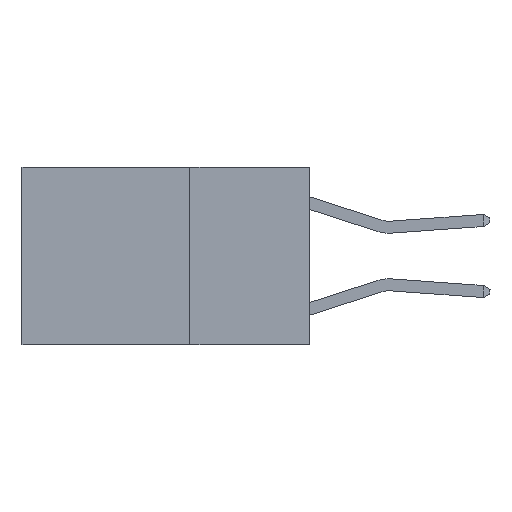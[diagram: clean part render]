
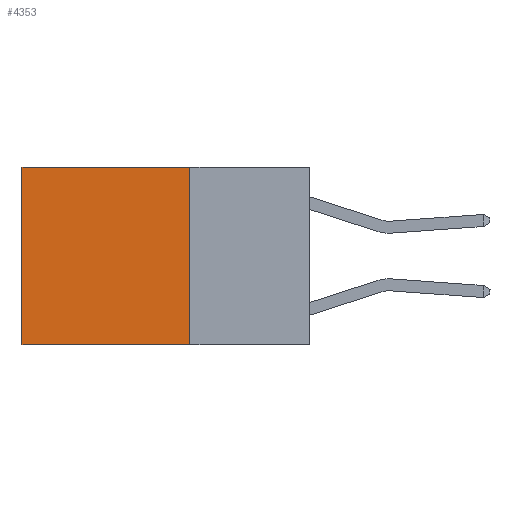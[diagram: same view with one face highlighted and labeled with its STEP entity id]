
A CAD part, left-side view. The second image highlights one B-rep face of the part: STEP entity #4353.
In plain terms, the highlighted planar face has unit normal (-1, 0, 0).
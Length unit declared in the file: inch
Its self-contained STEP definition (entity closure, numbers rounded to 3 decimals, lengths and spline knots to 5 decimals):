
#107 = EDGE_CURVE ( 'NONE', #16275, #7895, #18530, .T. ) ;
#217 = LINE ( 'NONE', #10510, #25759 ) ;
#487 = DIRECTION ( 'NONE',  ( 0., 0., -1. ) ) ;
#1403 = LINE ( 'NONE', #7564, #20456 ) ;
#2352 = CARTESIAN_POINT ( 'NONE',  ( 0.2625, 0.6, 0. ) ) ;
#2807 = PLANE ( 'NONE',  #22214 ) ;
#4353 = ADVANCED_FACE ( 'NONE', ( #18980 ), #2807, .F. ) ;
#5501 = EDGE_CURVE ( 'NONE', #7895, #13441, #10542, .T. ) ;
#6148 = ORIENTED_EDGE ( 'NONE', *, *, #22164, .T. ) ;
#6643 = DIRECTION ( 'NONE',  ( 0., 0., -1. ) ) ;
#7204 = CARTESIAN_POINT ( 'NONE',  ( 0.2625, 0.25, 0. ) ) ;
#7564 = CARTESIAN_POINT ( 'NONE',  ( 0.2625, 0.25, 0. ) ) ;
#7895 = VERTEX_POINT ( 'NONE', #25514 ) ;
#8438 = EDGE_CURVE ( 'NONE', #16275, #22133, #1403, .T. ) ;
#9659 = CARTESIAN_POINT ( 'NONE',  ( 0.2625, 0.25, 0. ) ) ;
#10442 = ORIENTED_EDGE ( 'NONE', *, *, #5501, .F. ) ;
#10510 = CARTESIAN_POINT ( 'NONE',  ( 0.2625, 0.6, 0. ) ) ;
#10542 = LINE ( 'NONE', #20313, #24118 ) ;
#11222 = DIRECTION ( 'NONE',  ( 0., 0., -1. ) ) ;
#11464 = ORIENTED_EDGE ( 'NONE', *, *, #8438, .T. ) ;
#12365 = CARTESIAN_POINT ( 'NONE',  ( 0.2625, 0.6, -0.37 ) ) ;
#12621 = ORIENTED_EDGE ( 'NONE', *, *, #107, .F. ) ;
#13109 = DIRECTION ( 'NONE',  ( 1., 0., 0. ) ) ;
#13441 = VERTEX_POINT ( 'NONE', #12365 ) ;
#15719 = DIRECTION ( 'NONE',  ( 0., 1., 0. ) ) ;
#16275 = VERTEX_POINT ( 'NONE', #9659 ) ;
#16313 = DIRECTION ( 'NONE',  ( 0., 1., 0. ) ) ;
#16434 = EDGE_LOOP ( 'NONE', ( #6148, #10442, #12621, #11464 ) ) ;
#18530 = LINE ( 'NONE', #18655, #19682 ) ;
#18655 = CARTESIAN_POINT ( 'NONE',  ( 0.2625, 0.25, 0. ) ) ;
#18980 = FACE_OUTER_BOUND ( 'NONE', #16434, .T. ) ;
#19682 = VECTOR ( 'NONE', #6643, 39.37008 ) ;
#20313 = CARTESIAN_POINT ( 'NONE',  ( 0.2625, 0.25, -0.37 ) ) ;
#20456 = VECTOR ( 'NONE', #15719, 39.37008 ) ;
#22133 = VERTEX_POINT ( 'NONE', #2352 ) ;
#22164 = EDGE_CURVE ( 'NONE', #22133, #13441, #217, .T. ) ;
#22214 = AXIS2_PLACEMENT_3D ( 'NONE', #7204, #13109, #11222 ) ;
#24118 = VECTOR ( 'NONE', #16313, 39.37008 ) ;
#25514 = CARTESIAN_POINT ( 'NONE',  ( 0.2625, 0.25, -0.37 ) ) ;
#25759 = VECTOR ( 'NONE', #487, 39.37008 ) ;
